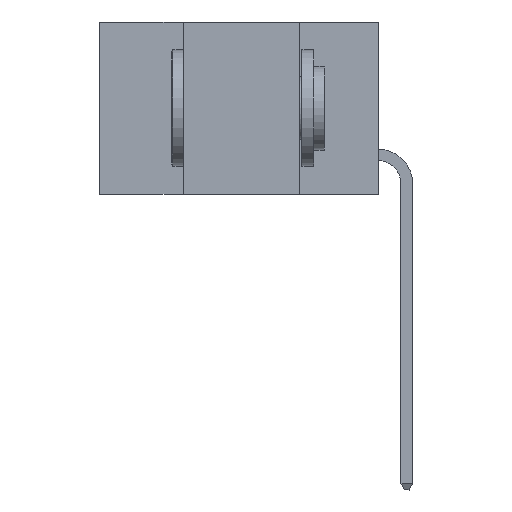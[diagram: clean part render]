
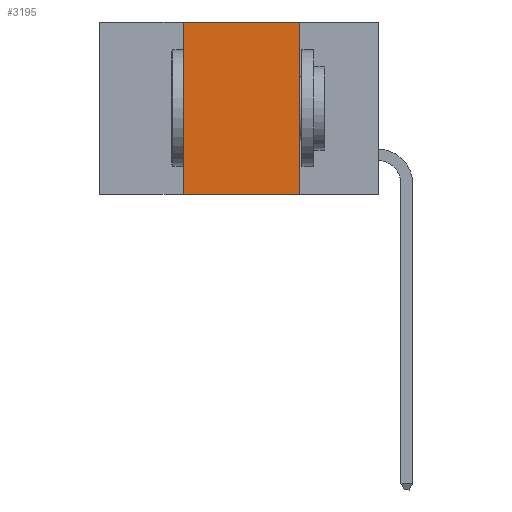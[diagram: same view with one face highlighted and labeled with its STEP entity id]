
A CAD part, left-side view. The second image highlights one B-rep face of the part: STEP entity #3195.
In plain terms, the highlighted planar face has unit normal (-1, 0, 0).
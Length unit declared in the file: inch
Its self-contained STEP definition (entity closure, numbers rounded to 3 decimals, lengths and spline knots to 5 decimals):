
#751 = EDGE_CURVE ( 'NONE', #6322, #17157, #20893, .T. ) ;
#898 = CARTESIAN_POINT ( 'NONE',  ( 0., 0.42, 0. ) ) ;
#3195 = ADVANCED_FACE ( 'NONE', ( #18714 ), #16367, .F. ) ;
#4256 = EDGE_CURVE ( 'NONE', #5118, #17157, #26601, .T. ) ;
#4916 = DIRECTION ( 'NONE',  ( 0., 0., -1. ) ) ;
#4942 = DIRECTION ( 'NONE',  ( 1., 0., 0. ) ) ;
#5088 = VECTOR ( 'NONE', #22207, 39.37008 ) ;
#5118 = VERTEX_POINT ( 'NONE', #23307 ) ;
#5955 = EDGE_LOOP ( 'NONE', ( #25327, #8230, #26350, #27469 ) ) ;
#6322 = VERTEX_POINT ( 'NONE', #20589 ) ;
#7039 = CARTESIAN_POINT ( 'NONE',  ( 0., 0.42, 0. ) ) ;
#8058 = CARTESIAN_POINT ( 'NONE',  ( 0., 0.6, 0. ) ) ;
#8230 = ORIENTED_EDGE ( 'NONE', *, *, #26336, .F. ) ;
#8883 = VECTOR ( 'NONE', #26167, 39.37008 ) ;
#11692 = CARTESIAN_POINT ( 'NONE',  ( 0., 0.17, 0. ) ) ;
#12833 = CARTESIAN_POINT ( 'NONE',  ( 0., 0.6, 0. ) ) ;
#12884 = EDGE_CURVE ( 'NONE', #5118, #20042, #27285, .T. ) ;
#14969 = DIRECTION ( 'NONE',  ( 0., -1., 0. ) ) ;
#15243 = VECTOR ( 'NONE', #20318, 39.37008 ) ;
#15815 = AXIS2_PLACEMENT_3D ( 'NONE', #8058, #4942, #4916 ) ;
#16367 = PLANE ( 'NONE',  #15815 ) ;
#17157 = VERTEX_POINT ( 'NONE', #23169 ) ;
#18714 = FACE_OUTER_BOUND ( 'NONE', #5955, .T. ) ;
#20042 = VERTEX_POINT ( 'NONE', #7039 ) ;
#20318 = DIRECTION ( 'NONE',  ( 0., 0., 1. ) ) ;
#20589 = CARTESIAN_POINT ( 'NONE',  ( 0., 0.17, 0. ) ) ;
#20893 = LINE ( 'NONE', #11692, #5088 ) ;
#21601 = LINE ( 'NONE', #12833, #26511 ) ;
#21984 = CARTESIAN_POINT ( 'NONE',  ( 0., 0.6, -0.37 ) ) ;
#22207 = DIRECTION ( 'NONE',  ( 0., 0., -1. ) ) ;
#23169 = CARTESIAN_POINT ( 'NONE',  ( 0., 0.17, -0.37 ) ) ;
#23307 = CARTESIAN_POINT ( 'NONE',  ( 0., 0.42, -0.37 ) ) ;
#25327 = ORIENTED_EDGE ( 'NONE', *, *, #751, .F. ) ;
#26167 = DIRECTION ( 'NONE',  ( 0., -1., 0. ) ) ;
#26336 = EDGE_CURVE ( 'NONE', #20042, #6322, #21601, .T. ) ;
#26350 = ORIENTED_EDGE ( 'NONE', *, *, #12884, .F. ) ;
#26511 = VECTOR ( 'NONE', #14969, 39.37008 ) ;
#26601 = LINE ( 'NONE', #21984, #8883 ) ;
#27285 = LINE ( 'NONE', #898, #15243 ) ;
#27469 = ORIENTED_EDGE ( 'NONE', *, *, #4256, .T. ) ;
